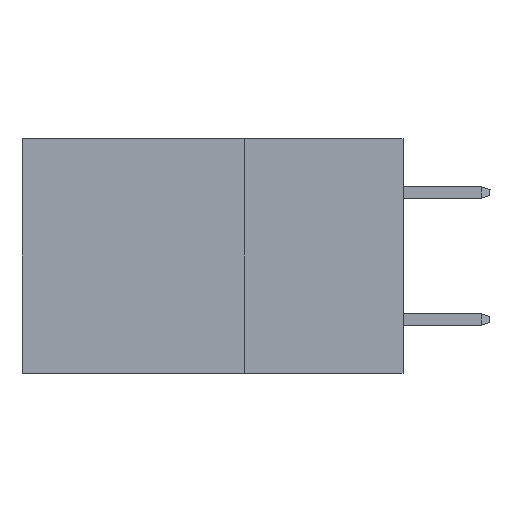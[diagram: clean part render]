
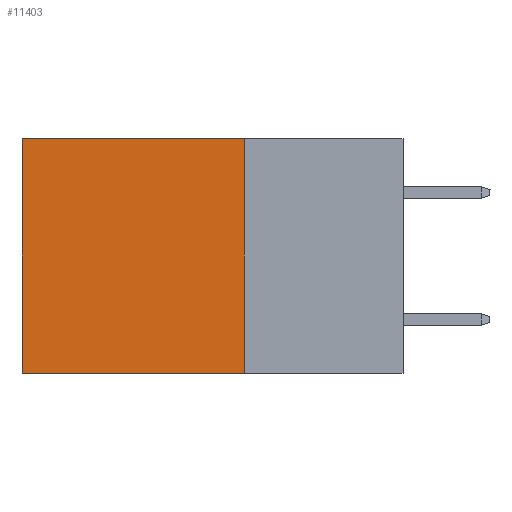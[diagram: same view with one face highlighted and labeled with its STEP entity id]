
A CAD part, left-side view. The second image highlights one B-rep face of the part: STEP entity #11403.
In plain terms, the highlighted planar face has unit normal (-1, 0, 0).
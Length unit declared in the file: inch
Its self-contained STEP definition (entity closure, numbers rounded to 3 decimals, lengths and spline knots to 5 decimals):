
#170 = EDGE_CURVE ( 'NONE', #14234, #26459, #3704, .T. ) ;
#242 = DIRECTION ( 'NONE',  ( 1., 0., 0. ) ) ;
#529 = CARTESIAN_POINT ( 'NONE',  ( 0.2875, 0.25, 0. ) ) ;
#1772 = VECTOR ( 'NONE', #19482, 39.37008 ) ;
#2189 = DIRECTION ( 'NONE',  ( 0., 0., -1. ) ) ;
#3030 = DIRECTION ( 'NONE',  ( 0., 0., -1. ) ) ;
#3256 = ORIENTED_EDGE ( 'NONE', *, *, #7178, .F. ) ;
#3421 = DIRECTION ( 'NONE',  ( 0., 1., 0. ) ) ;
#3704 = LINE ( 'NONE', #28347, #1772 ) ;
#4396 = LINE ( 'NONE', #14091, #10550 ) ;
#7178 = EDGE_CURVE ( 'NONE', #20580, #28008, #23498, .T. ) ;
#8683 = EDGE_LOOP ( 'NONE', ( #20453, #3256, #19673, #22543 ) ) ;
#10550 = VECTOR ( 'NONE', #3030, 39.37008 ) ;
#10725 = EDGE_CURVE ( 'NONE', #26459, #28008, #21424, .T. ) ;
#10868 = AXIS2_PLACEMENT_3D ( 'NONE', #529, #242, #2189 ) ;
#11403 = ADVANCED_FACE ( 'NONE', ( #20311 ), #20741, .F. ) ;
#12729 = CARTESIAN_POINT ( 'NONE',  ( 0.2875, 0.6, 0. ) ) ;
#12811 = CARTESIAN_POINT ( 'NONE',  ( 0.2875, 0.6, 0. ) ) ;
#14091 = CARTESIAN_POINT ( 'NONE',  ( 0.2875, 0.25, 0. ) ) ;
#14234 = VERTEX_POINT ( 'NONE', #16355 ) ;
#15040 = VECTOR ( 'NONE', #15066, 39.37008 ) ;
#15066 = DIRECTION ( 'NONE',  ( 0., 0., -1. ) ) ;
#16355 = CARTESIAN_POINT ( 'NONE',  ( 0.2875, 0.25, 0. ) ) ;
#18121 = CARTESIAN_POINT ( 'NONE',  ( 0.2875, 0.25, -0.37 ) ) ;
#18904 = CARTESIAN_POINT ( 'NONE',  ( 0.2875, 0.25, -0.37 ) ) ;
#19482 = DIRECTION ( 'NONE',  ( 0., 1., 0. ) ) ;
#19673 = ORIENTED_EDGE ( 'NONE', *, *, #24828, .F. ) ;
#20183 = CARTESIAN_POINT ( 'NONE',  ( 0.2875, 0.6, -0.37 ) ) ;
#20311 = FACE_OUTER_BOUND ( 'NONE', #8683, .T. ) ;
#20453 = ORIENTED_EDGE ( 'NONE', *, *, #10725, .T. ) ;
#20580 = VERTEX_POINT ( 'NONE', #18121 ) ;
#20741 = PLANE ( 'NONE',  #10868 ) ;
#21424 = LINE ( 'NONE', #12729, #15040 ) ;
#22543 = ORIENTED_EDGE ( 'NONE', *, *, #170, .T. ) ;
#22718 = VECTOR ( 'NONE', #3421, 39.37008 ) ;
#23498 = LINE ( 'NONE', #18904, #22718 ) ;
#24828 = EDGE_CURVE ( 'NONE', #14234, #20580, #4396, .T. ) ;
#26459 = VERTEX_POINT ( 'NONE', #12811 ) ;
#28008 = VERTEX_POINT ( 'NONE', #20183 ) ;
#28347 = CARTESIAN_POINT ( 'NONE',  ( 0.2875, 0.25, 0. ) ) ;
